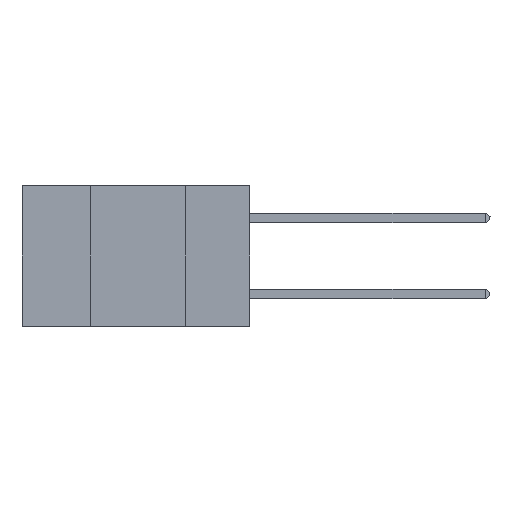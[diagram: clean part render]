
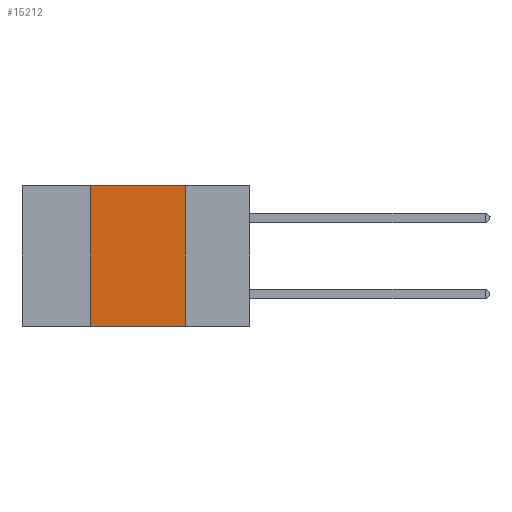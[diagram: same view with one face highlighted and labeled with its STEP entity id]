
A CAD part, left-side view. The second image highlights one B-rep face of the part: STEP entity #15212.
In plain terms, the highlighted planar face has unit normal (-1, 0, 0).
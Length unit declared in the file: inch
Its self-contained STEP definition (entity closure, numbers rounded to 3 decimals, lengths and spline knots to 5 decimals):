
#136 = DIRECTION ( 'NONE',  ( 1., 0., 0. ) ) ;
#1031 = LINE ( 'NONE', #5535, #24934 ) ;
#1890 = ORIENTED_EDGE ( 'NONE', *, *, #8609, .T. ) ;
#3664 = LINE ( 'NONE', #10349, #5562 ) ;
#4204 = AXIS2_PLACEMENT_3D ( 'NONE', #12328, #136, #14522 ) ;
#4249 = ORIENTED_EDGE ( 'NONE', *, *, #9834, .F. ) ;
#5535 = CARTESIAN_POINT ( 'NONE',  ( 0., 0.17, 0. ) ) ;
#5562 = VECTOR ( 'NONE', #25040, 39.37008 ) ;
#5738 = ORIENTED_EDGE ( 'NONE', *, *, #25997, .F. ) ;
#5844 = DIRECTION ( 'NONE',  ( 0., -1., 0. ) ) ;
#6142 = FACE_OUTER_BOUND ( 'NONE', #7737, .T. ) ;
#7273 = VERTEX_POINT ( 'NONE', #19042 ) ;
#7737 = EDGE_LOOP ( 'NONE', ( #8031, #4249, #5738, #1890 ) ) ;
#8031 = ORIENTED_EDGE ( 'NONE', *, *, #11427, .F. ) ;
#8046 = PLANE ( 'NONE',  #4204 ) ;
#8461 = VERTEX_POINT ( 'NONE', #23797 ) ;
#8609 = EDGE_CURVE ( 'NONE', #9174, #15403, #11880, .T. ) ;
#9174 = VERTEX_POINT ( 'NONE', #21403 ) ;
#9834 = EDGE_CURVE ( 'NONE', #7273, #8461, #3664, .T. ) ;
#10349 = CARTESIAN_POINT ( 'NONE',  ( 0., 0.6, 0. ) ) ;
#10975 = LINE ( 'NONE', #21781, #14318 ) ;
#11053 = CARTESIAN_POINT ( 'NONE',  ( 0., 0.17, -0.37 ) ) ;
#11427 = EDGE_CURVE ( 'NONE', #8461, #15403, #1031, .T. ) ;
#11880 = LINE ( 'NONE', #26933, #15481 ) ;
#12328 = CARTESIAN_POINT ( 'NONE',  ( 0., 0.6, 0. ) ) ;
#14318 = VECTOR ( 'NONE', #23846, 39.37008 ) ;
#14522 = DIRECTION ( 'NONE',  ( 0., 0., -1. ) ) ;
#15212 = ADVANCED_FACE ( 'NONE', ( #6142 ), #8046, .F. ) ;
#15403 = VERTEX_POINT ( 'NONE', #11053 ) ;
#15481 = VECTOR ( 'NONE', #5844, 39.37008 ) ;
#15538 = DIRECTION ( 'NONE',  ( 0., 0., -1. ) ) ;
#19042 = CARTESIAN_POINT ( 'NONE',  ( 0., 0.42, 0. ) ) ;
#21403 = CARTESIAN_POINT ( 'NONE',  ( 0., 0.42, -0.37 ) ) ;
#21781 = CARTESIAN_POINT ( 'NONE',  ( 0., 0.42, 0. ) ) ;
#23797 = CARTESIAN_POINT ( 'NONE',  ( 0., 0.17, 0. ) ) ;
#23846 = DIRECTION ( 'NONE',  ( 0., 0., 1. ) ) ;
#24934 = VECTOR ( 'NONE', #15538, 39.37008 ) ;
#25040 = DIRECTION ( 'NONE',  ( 0., -1., 0. ) ) ;
#25997 = EDGE_CURVE ( 'NONE', #9174, #7273, #10975, .T. ) ;
#26933 = CARTESIAN_POINT ( 'NONE',  ( 0., 0.6, -0.37 ) ) ;
